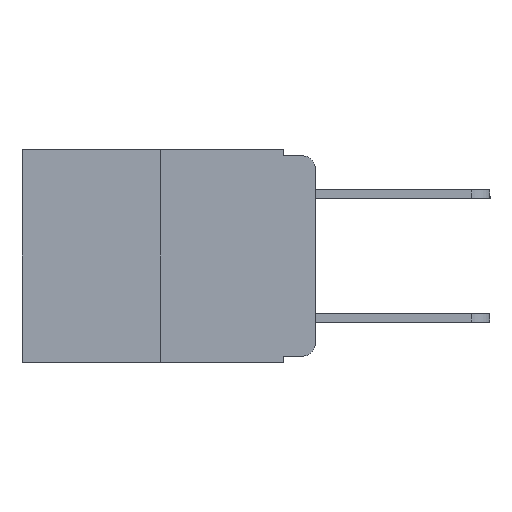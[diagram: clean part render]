
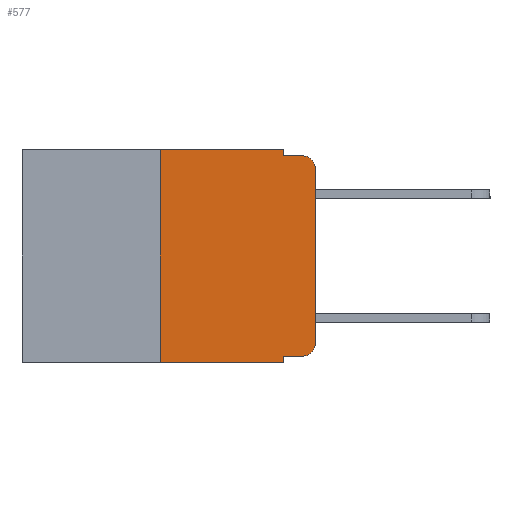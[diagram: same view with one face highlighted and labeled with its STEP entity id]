
A CAD part, left-side view. The second image highlights one B-rep face of the part: STEP entity #577.
In plain terms, the highlighted planar face has unit normal (-1, 0, 0).
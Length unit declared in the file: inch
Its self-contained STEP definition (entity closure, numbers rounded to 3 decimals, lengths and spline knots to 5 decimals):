
#6 = CARTESIAN_POINT ( 'NONE',  ( 0., 0.02, -0.313 ) ) ;
#54 = CARTESIAN_POINT ( 'NONE',  ( 0., 0.02, -0.01 ) ) ;
#57 = LINE ( 'NONE', #3598, #18058 ) ;
#468 = LINE ( 'NONE', #10018, #18349 ) ;
#577 = ADVANCED_FACE ( 'NONE', ( #19275 ), #19879, .F. ) ;
#833 = VECTOR ( 'NONE', #13578, 39.37008 ) ;
#851 = CARTESIAN_POINT ( 'NONE',  ( 0., 0.051, -0.01 ) ) ;
#1700 = CIRCLE ( 'NONE', #6847, 0.02 ) ;
#2193 = DIRECTION ( 'NONE',  ( 0., 0., -1. ) ) ;
#2688 = CARTESIAN_POINT ( 'NONE',  ( 0., 0.25, -0.343 ) ) ;
#3357 = DIRECTION ( 'NONE',  ( 0., -1., 0. ) ) ;
#3598 = CARTESIAN_POINT ( 'NONE',  ( 0., 0.051, 0. ) ) ;
#3829 = VERTEX_POINT ( 'NONE', #19937 ) ;
#3992 = EDGE_LOOP ( 'NONE', ( #7589, #7414, #7390, #6406, #7198, #5475, #5207, #4035, #4008, #18452 ) ) ;
#4008 = ORIENTED_EDGE ( 'NONE', *, *, #13456, .T. ) ;
#4035 = ORIENTED_EDGE ( 'NONE', *, *, #12218, .F. ) ;
#4260 = VECTOR ( 'NONE', #16607, 39.37008 ) ;
#4760 = CARTESIAN_POINT ( 'NONE',  ( 0., 0., 0. ) ) ;
#4793 = DIRECTION ( 'NONE',  ( 0., -1., 0. ) ) ;
#5044 = VECTOR ( 'NONE', #3357, 39.37008 ) ;
#5207 = ORIENTED_EDGE ( 'NONE', *, *, #19725, .T. ) ;
#5401 = AXIS2_PLACEMENT_3D ( 'NONE', #6, #12678, #2193 ) ;
#5475 = ORIENTED_EDGE ( 'NONE', *, *, #12766, .F. ) ;
#6009 = EDGE_CURVE ( 'NONE', #7801, #12447, #1700, .T. ) ;
#6406 = ORIENTED_EDGE ( 'NONE', *, *, #20469, .F. ) ;
#6503 = DIRECTION ( 'NONE',  ( 0., 0., 1. ) ) ;
#6532 = CIRCLE ( 'NONE', #5401, 0.02 ) ;
#6558 = CARTESIAN_POINT ( 'NONE',  ( 0., 0.25, 0. ) ) ;
#6677 = DIRECTION ( 'NONE',  ( -1., 0., 0. ) ) ;
#6847 = AXIS2_PLACEMENT_3D ( 'NONE', #16731, #6677, #18294 ) ;
#7198 = ORIENTED_EDGE ( 'NONE', *, *, #8011, .F. ) ;
#7390 = ORIENTED_EDGE ( 'NONE', *, *, #18247, .F. ) ;
#7414 = ORIENTED_EDGE ( 'NONE', *, *, #6009, .T. ) ;
#7484 = EDGE_CURVE ( 'NONE', #19063, #13530, #6532, .T. ) ;
#7564 = VERTEX_POINT ( 'NONE', #14394 ) ;
#7589 = ORIENTED_EDGE ( 'NONE', *, *, #21705, .T. ) ;
#7801 = VERTEX_POINT ( 'NONE', #18700 ) ;
#8011 = EDGE_CURVE ( 'NONE', #8742, #17905, #10106, .T. ) ;
#8491 = VECTOR ( 'NONE', #6503, 39.37008 ) ;
#8742 = VERTEX_POINT ( 'NONE', #11977 ) ;
#9105 = VERTEX_POINT ( 'NONE', #2688 ) ;
#9734 = LINE ( 'NONE', #10426, #5044 ) ;
#10018 = CARTESIAN_POINT ( 'NONE',  ( 0., 0.473, -0.343 ) ) ;
#10025 = VERTEX_POINT ( 'NONE', #13141 ) ;
#10106 = LINE ( 'NONE', #20694, #13940 ) ;
#10426 = CARTESIAN_POINT ( 'NONE',  ( 0., 0.051, -0.333 ) ) ;
#10512 = DIRECTION ( 'NONE',  ( 0., 0., -1. ) ) ;
#11174 = DIRECTION ( 'NONE',  ( 0., -1., 0. ) ) ;
#11298 = AXIS2_PLACEMENT_3D ( 'NONE', #21171, #21025, #20900 ) ;
#11977 = CARTESIAN_POINT ( 'NONE',  ( 0., 0.25, 0. ) ) ;
#12218 = EDGE_CURVE ( 'NONE', #3829, #10025, #17680, .T. ) ;
#12447 = VERTEX_POINT ( 'NONE', #54 ) ;
#12678 = DIRECTION ( 'NONE',  ( -1., 0., 0. ) ) ;
#12766 = EDGE_CURVE ( 'NONE', #9105, #8742, #12856, .T. ) ;
#12856 = LINE ( 'NONE', #6558, #4260 ) ;
#12877 = VECTOR ( 'NONE', #10512, 39.37008 ) ;
#13141 = CARTESIAN_POINT ( 'NONE',  ( 0., 0.051, -0.343 ) ) ;
#13456 = EDGE_CURVE ( 'NONE', #3829, #19063, #9734, .T. ) ;
#13530 = VERTEX_POINT ( 'NONE', #17094 ) ;
#13578 = DIRECTION ( 'NONE',  ( 0., -1., 0. ) ) ;
#13940 = VECTOR ( 'NONE', #11174, 39.37008 ) ;
#14394 = CARTESIAN_POINT ( 'NONE',  ( 0., 0.051, -0.01 ) ) ;
#15207 = CARTESIAN_POINT ( 'NONE',  ( 0., 0.02, -0.333 ) ) ;
#15551 = DIRECTION ( 'NONE',  ( 0., 0., -1. ) ) ;
#16607 = DIRECTION ( 'NONE',  ( 0., 0., 1. ) ) ;
#16731 = CARTESIAN_POINT ( 'NONE',  ( 0., 0.02, -0.03 ) ) ;
#17094 = CARTESIAN_POINT ( 'NONE',  ( 0., 0., -0.313 ) ) ;
#17340 = CARTESIAN_POINT ( 'NONE',  ( 0., 0.051, 0. ) ) ;
#17680 = LINE ( 'NONE', #18553, #12877 ) ;
#17905 = VERTEX_POINT ( 'NONE', #17340 ) ;
#18058 = VECTOR ( 'NONE', #15551, 39.37008 ) ;
#18247 = EDGE_CURVE ( 'NONE', #7564, #12447, #18627, .T. ) ;
#18294 = DIRECTION ( 'NONE',  ( 0., 0., -1. ) ) ;
#18349 = VECTOR ( 'NONE', #4793, 39.37008 ) ;
#18452 = ORIENTED_EDGE ( 'NONE', *, *, #7484, .T. ) ;
#18553 = CARTESIAN_POINT ( 'NONE',  ( 0., 0.051, 0. ) ) ;
#18627 = LINE ( 'NONE', #851, #833 ) ;
#18700 = CARTESIAN_POINT ( 'NONE',  ( 0., 0., -0.03 ) ) ;
#19063 = VERTEX_POINT ( 'NONE', #15207 ) ;
#19275 = FACE_OUTER_BOUND ( 'NONE', #3992, .T. ) ;
#19725 = EDGE_CURVE ( 'NONE', #9105, #10025, #468, .T. ) ;
#19879 = PLANE ( 'NONE',  #11298 ) ;
#19937 = CARTESIAN_POINT ( 'NONE',  ( 0., 0.051, -0.333 ) ) ;
#20469 = EDGE_CURVE ( 'NONE', #17905, #7564, #57, .T. ) ;
#20694 = CARTESIAN_POINT ( 'NONE',  ( 0., 0.473, 0. ) ) ;
#20900 = DIRECTION ( 'NONE',  ( 0., 0., -1. ) ) ;
#21025 = DIRECTION ( 'NONE',  ( 1., 0., 0. ) ) ;
#21171 = CARTESIAN_POINT ( 'NONE',  ( 0., 0.473, 0. ) ) ;
#21350 = LINE ( 'NONE', #4760, #8491 ) ;
#21705 = EDGE_CURVE ( 'NONE', #13530, #7801, #21350, .T. ) ;
